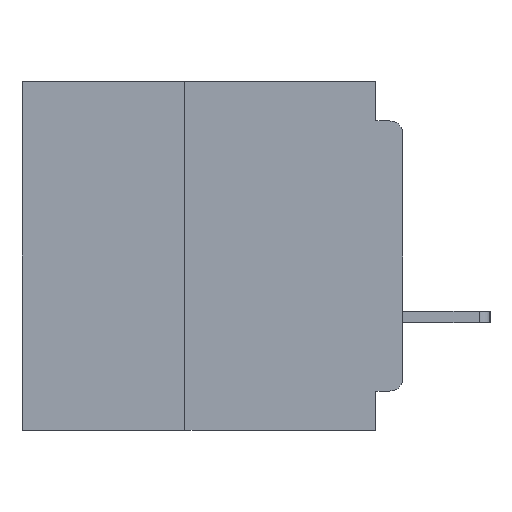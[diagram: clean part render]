
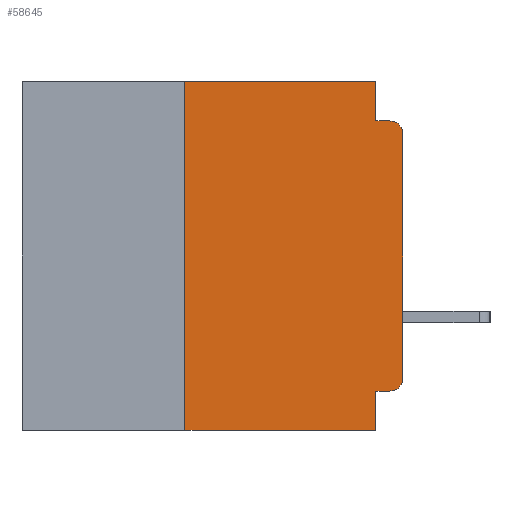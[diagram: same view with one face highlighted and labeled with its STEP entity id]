
A CAD part, left-side view. The second image highlights one B-rep face of the part: STEP entity #58645.
In plain terms, the highlighted planar face has unit normal (-1, 0, 0).
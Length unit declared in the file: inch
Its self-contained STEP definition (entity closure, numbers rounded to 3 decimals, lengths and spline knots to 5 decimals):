
#349 = DIRECTION ( 'NONE',  ( 0., 0., -1. ) ) ;
#713 = CIRCLE ( 'NONE', #50563, 0.015 ) ;
#2970 = EDGE_CURVE ( 'NONE', #64184, #60500, #45283, .T. ) ;
#3493 = ORIENTED_EDGE ( 'NONE', *, *, #8417, .F. ) ;
#4263 = ORIENTED_EDGE ( 'NONE', *, *, #62897, .F. ) ;
#5078 = AXIS2_PLACEMENT_3D ( 'NONE', #16955, #27077, #61464 ) ;
#5674 = DIRECTION ( 'NONE',  ( 0., 0., -1. ) ) ;
#6272 = CARTESIAN_POINT ( 'NONE',  ( 0., 0.015, -0.06 ) ) ;
#6794 = VECTOR ( 'NONE', #41842, 39.37008 ) ;
#7064 = DIRECTION ( 'NONE',  ( 0., 0., -1. ) ) ;
#8417 = EDGE_CURVE ( 'NONE', #52306, #11716, #29347, .T. ) ;
#9582 = VERTEX_POINT ( 'NONE', #45801 ) ;
#10233 = ORIENTED_EDGE ( 'NONE', *, *, #51414, .T. ) ;
#10832 = VECTOR ( 'NONE', #62224, 39.37008 ) ;
#11284 = DIRECTION ( 'NONE',  ( 0., 0., -1. ) ) ;
#11484 = VECTOR ( 'NONE', #20340, 39.37008 ) ;
#11716 = VERTEX_POINT ( 'NONE', #61279 ) ;
#11761 = CARTESIAN_POINT ( 'NONE',  ( 0., 0., -0.06 ) ) ;
#11872 = CARTESIAN_POINT ( 'NONE',  ( 0., 0.031, -0.4 ) ) ;
#16247 = ORIENTED_EDGE ( 'NONE', *, *, #2970, .T. ) ;
#16712 = VERTEX_POINT ( 'NONE', #33442 ) ;
#16955 = CARTESIAN_POINT ( 'NONE',  ( 0., 0.437, 0. ) ) ;
#17109 = AXIS2_PLACEMENT_3D ( 'NONE', #6272, #41137, #11284 ) ;
#17710 = CARTESIAN_POINT ( 'NONE',  ( 0., 0., -0.355 ) ) ;
#17794 = VECTOR ( 'NONE', #32228, 39.37008 ) ;
#20340 = DIRECTION ( 'NONE',  ( 0., -1., 0. ) ) ;
#20665 = CARTESIAN_POINT ( 'NONE',  ( 0., 0.031, -0.4 ) ) ;
#21295 = ORIENTED_EDGE ( 'NONE', *, *, #28209, .T. ) ;
#23088 = ORIENTED_EDGE ( 'NONE', *, *, #26578, .F. ) ;
#24139 = LINE ( 'NONE', #17710, #10832 ) ;
#25722 = EDGE_CURVE ( 'NONE', #60500, #58154, #50568, .T. ) ;
#26048 = ORIENTED_EDGE ( 'NONE', *, *, #35889, .F. ) ;
#26051 = LINE ( 'NONE', #41115, #63761 ) ;
#26140 = DIRECTION ( 'NONE',  ( 0., 0., 1. ) ) ;
#26578 = EDGE_CURVE ( 'NONE', #39630, #50830, #24139, .T. ) ;
#27077 = DIRECTION ( 'NONE',  ( 1., 0., 0. ) ) ;
#27083 = CARTESIAN_POINT ( 'NONE',  ( 0., 0., -0.34 ) ) ;
#27205 = CARTESIAN_POINT ( 'NONE',  ( 0., 0., -0.045 ) ) ;
#27469 = VECTOR ( 'NONE', #54178, 39.37008 ) ;
#27797 = VECTOR ( 'NONE', #5674, 39.37008 ) ;
#28209 = EDGE_CURVE ( 'NONE', #16712, #62826, #64076, .T. ) ;
#29347 = LINE ( 'NONE', #30613, #27797 ) ;
#29608 = EDGE_CURVE ( 'NONE', #50830, #62826, #41022, .T. ) ;
#30362 = DIRECTION ( 'NONE',  ( -1., 0., 0. ) ) ;
#30443 = CARTESIAN_POINT ( 'NONE',  ( 0., 0.031, -0.355 ) ) ;
#30582 = ORIENTED_EDGE ( 'NONE', *, *, #29608, .F. ) ;
#30613 = CARTESIAN_POINT ( 'NONE',  ( 0., 0.031, 0. ) ) ;
#31159 = ORIENTED_EDGE ( 'NONE', *, *, #35307, .F. ) ;
#31846 = LINE ( 'NONE', #32158, #6794 ) ;
#32138 = ORIENTED_EDGE ( 'NONE', *, *, #25722, .T. ) ;
#32158 = CARTESIAN_POINT ( 'NONE',  ( 0., 0.437, 0. ) ) ;
#32228 = DIRECTION ( 'NONE',  ( 0., -1., 0. ) ) ;
#32229 = CARTESIAN_POINT ( 'NONE',  ( 0., 0.015, -0.355 ) ) ;
#32776 = EDGE_LOOP ( 'NONE', ( #16247, #32138, #31159, #3493, #26048, #4263, #21295, #30582, #23088, #10233 ) ) ;
#33442 = CARTESIAN_POINT ( 'NONE',  ( 0., 0.25, -0.4 ) ) ;
#35307 = EDGE_CURVE ( 'NONE', #11716, #58154, #42722, .T. ) ;
#35889 = EDGE_CURVE ( 'NONE', #9582, #52306, #31846, .T. ) ;
#39630 = VERTEX_POINT ( 'NONE', #32229 ) ;
#40160 = CARTESIAN_POINT ( 'NONE',  ( 0., 0.437, -0.4 ) ) ;
#40559 = FACE_OUTER_BOUND ( 'NONE', #32776, .T. ) ;
#41022 = LINE ( 'NONE', #11872, #54060 ) ;
#41115 = CARTESIAN_POINT ( 'NONE',  ( 0., 0.25, -0.4 ) ) ;
#41137 = DIRECTION ( 'NONE',  ( -1., 0., 0. ) ) ;
#41842 = DIRECTION ( 'NONE',  ( 0., -1., 0. ) ) ;
#42722 = LINE ( 'NONE', #27205, #17794 ) ;
#45283 = LINE ( 'NONE', #49248, #27469 ) ;
#45801 = CARTESIAN_POINT ( 'NONE',  ( 0., 0.25, 0. ) ) ;
#49248 = CARTESIAN_POINT ( 'NONE',  ( 0., 0., 0. ) ) ;
#50563 = AXIS2_PLACEMENT_3D ( 'NONE', #59782, #30362, #349 ) ;
#50568 = CIRCLE ( 'NONE', #17109, 0.015 ) ;
#50830 = VERTEX_POINT ( 'NONE', #30443 ) ;
#51414 = EDGE_CURVE ( 'NONE', #39630, #64184, #713, .T. ) ;
#52306 = VERTEX_POINT ( 'NONE', #57790 ) ;
#54060 = VECTOR ( 'NONE', #7064, 39.37008 ) ;
#54178 = DIRECTION ( 'NONE',  ( 0., 0., 1. ) ) ;
#56374 = PLANE ( 'NONE',  #5078 ) ;
#57790 = CARTESIAN_POINT ( 'NONE',  ( 0., 0.031, 0. ) ) ;
#58154 = VERTEX_POINT ( 'NONE', #61309 ) ;
#58645 = ADVANCED_FACE ( 'NONE', ( #40559 ), #56374, .F. ) ;
#59782 = CARTESIAN_POINT ( 'NONE',  ( 0., 0.015, -0.34 ) ) ;
#60500 = VERTEX_POINT ( 'NONE', #11761 ) ;
#61279 = CARTESIAN_POINT ( 'NONE',  ( 0., 0.031, -0.045 ) ) ;
#61309 = CARTESIAN_POINT ( 'NONE',  ( 0., 0.015, -0.045 ) ) ;
#61464 = DIRECTION ( 'NONE',  ( 0., 0., -1. ) ) ;
#62224 = DIRECTION ( 'NONE',  ( 0., 1., 0. ) ) ;
#62826 = VERTEX_POINT ( 'NONE', #20665 ) ;
#62897 = EDGE_CURVE ( 'NONE', #16712, #9582, #26051, .T. ) ;
#63761 = VECTOR ( 'NONE', #26140, 39.37008 ) ;
#64076 = LINE ( 'NONE', #40160, #11484 ) ;
#64184 = VERTEX_POINT ( 'NONE', #27083 ) ;
